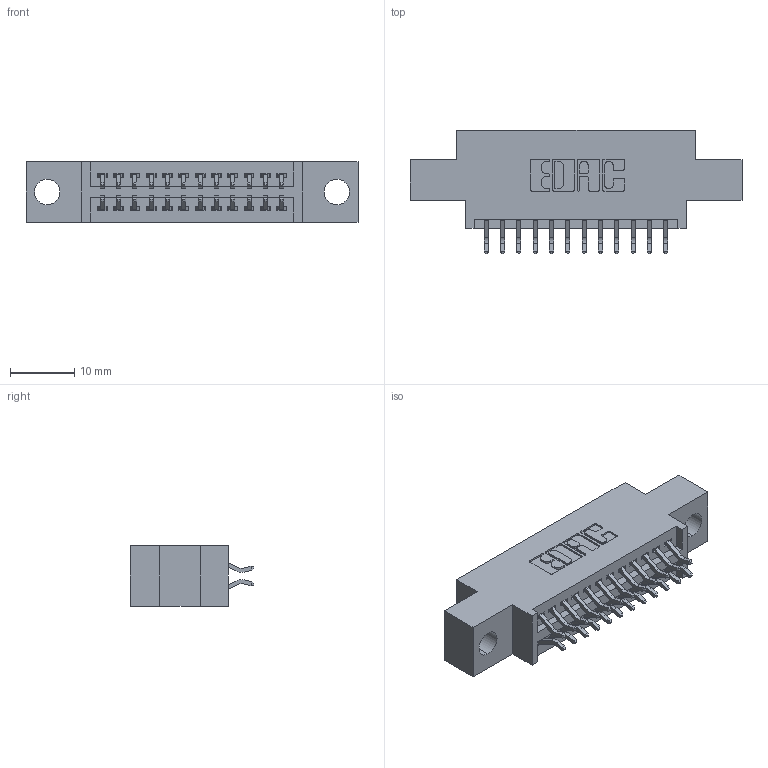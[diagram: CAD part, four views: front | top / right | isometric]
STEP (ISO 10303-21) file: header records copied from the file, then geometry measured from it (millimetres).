
FILE_DESCRIPTION (( 'STEP AP203' ), '1' );
FILE_NAME ('345-024-556-804.STEP', '2021-05-19T22:32:34', ( '' ), ( '' ), 'SwSTEP 2.0', 'SolidWorks 2020', '' );
FILE_SCHEMA (( 'CONFIG_CONTROL_DESIGN' ));
Length unit declared in the file: inch
Products named in the file (3): 345-292-001_556 Tail; 345-024-556-804; 345 Part_0.170 Offset - 0.156 Dia-TI
Assembly tree (25 placements, depth 2):
  345-024-556-804
    345 Part_0.170 Offset - 0.156 Dia-TI
    345-292-001_556 Tail  x24
Bounding box: 51.69 x 19.24 x 9.4 mm (x, y, z)
Volume: 4522.4 mm3; surface area: 6077.8 mm2
Topology: 25 solids, 25 shells, 1488 faces, 4397 edges, 2898 vertices
Faces by surface type: plane 986, cylinder 502
Entity records: 14225 total; most frequent: CARTESIAN_POINT 2434, ORIENTED_EDGE 2354, DIRECTION 2169, EDGE_CURVE 1177, VECTOR 989, LINE 989, VERTEX_POINT 782, AXIS2_PLACEMENT_3D 590
